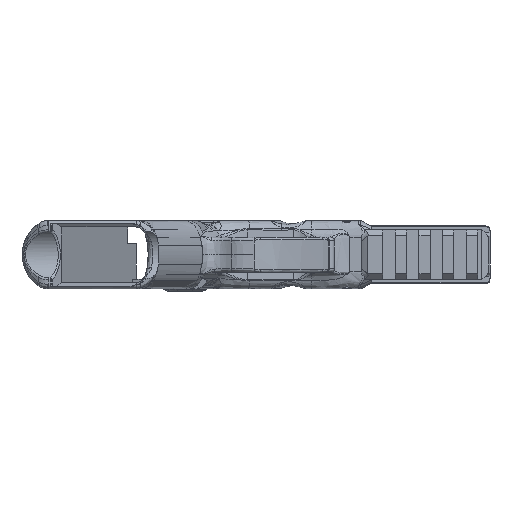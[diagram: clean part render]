
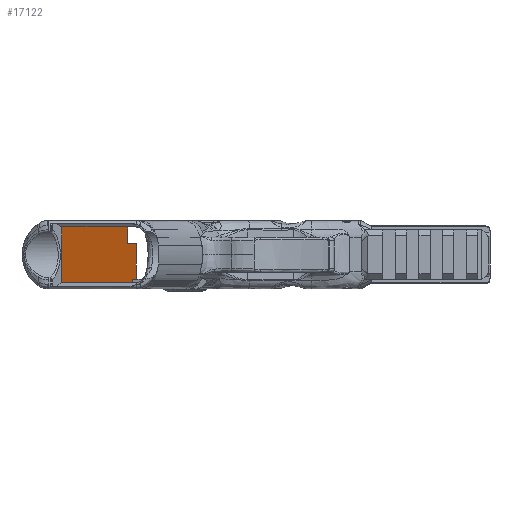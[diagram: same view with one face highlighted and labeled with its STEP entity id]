
A CAD part, front view. The second image highlights one B-rep face of the part: STEP entity #17122.
In plain terms, the highlighted planar face has unit normal (0.951, -0.309, 0).
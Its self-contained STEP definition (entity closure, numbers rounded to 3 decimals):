
#207 = ORIENTED_EDGE ( 'NONE', *, *, #1943, .F. ) ;
#595 = CARTESIAN_POINT ( 'NONE',  ( 2.237, -97.997, -11.765 ) ) ;
#730 = EDGE_CURVE ( 'NONE', #10152, #47471, #28344, .T. ) ;
#1692 = CARTESIAN_POINT ( 'NONE',  ( 33.591, -1.5, 4.75 ) ) ;
#1943 = EDGE_CURVE ( 'NONE', #28863, #14634, #2948, .T. ) ;
#2087 = CARTESIAN_POINT ( 'NONE',  ( 33.591, -1.5, -5.875 ) ) ;
#2320 = CARTESIAN_POINT ( 'NONE',  ( 18.86, -46.836, 4.75 ) ) ;
#2919 = CARTESIAN_POINT ( 'NONE',  ( 32.169, -5.875, -10.375 ) ) ;
#2948 =( BOUNDED_CURVE ( )  B_SPLINE_CURVE ( 3, ( #43225, #15098, #47478, #41535 ),
 .UNSPECIFIED., .F., .F. ) 
 B_SPLINE_CURVE_WITH_KNOTS ( ( 4, 4 ),
 ( 1.395, 1.571 ),
 .UNSPECIFIED. ) 
 CURVE ( )  GEOMETRIC_REPRESENTATION_ITEM ( )  RATIONAL_B_SPLINE_CURVE ( ( 1., 0.997, 0.997, 1. ) ) 
 REPRESENTATION_ITEM ( '' )  );
#3524 = DIRECTION ( 'NONE',  ( -0.951, 0.309, 0. ) ) ;
#3628 = VERTEX_POINT ( 'NONE', #1692 ) ;
#5233 = VECTOR ( 'NONE', #49592, 1000. ) ;
#6991 = PLANE ( 'NONE',  #35532 ) ;
#7092 = VECTOR ( 'NONE', #26142, 1000. ) ;
#7588 = VECTOR ( 'NONE', #37738, 1000. ) ;
#7966 = CARTESIAN_POINT ( 'NONE',  ( 32.169, -5.875, -11.75 ) ) ;
#8550 = CARTESIAN_POINT ( 'NONE',  ( 2.256, -97.94, -11.755 ) ) ;
#8653 =( BOUNDED_CURVE ( )  B_SPLINE_CURVE ( 3, ( #23826, #12148, #40541, #45031 ),
 .UNSPECIFIED., .F., .F. ) 
 B_SPLINE_CURVE_WITH_KNOTS ( ( 4, 4 ),
 ( 4.888, 4.891 ),
 .UNSPECIFIED. ) 
 CURVE ( )  GEOMETRIC_REPRESENTATION_ITEM ( )  RATIONAL_B_SPLINE_CURVE ( ( 1., 1., 1., 1. ) ) 
 REPRESENTATION_ITEM ( '' )  );
#10152 = VERTEX_POINT ( 'NONE', #47347 ) ;
#10278 = LINE ( 'NONE', #2087, #29029 ) ;
#10696 = LINE ( 'NONE', #39086, #15399 ) ;
#10897 = ORIENTED_EDGE ( 'NONE', *, *, #45271, .T. ) ;
#10984 = VERTEX_POINT ( 'NONE', #22116 ) ;
#12148 = CARTESIAN_POINT ( 'NONE',  ( 2.236, -97.998, -11.766 ) ) ;
#13134 = LINE ( 'NONE', #41264, #7092 ) ;
#13365 = EDGE_CURVE ( 'NONE', #47471, #16325, #8653, .T. ) ;
#13889 =( BOUNDED_CURVE ( )  B_SPLINE_CURVE ( 3, ( #15627, #19864, #15879, #28092 ),
 .UNSPECIFIED., .F., .T. ) 
 B_SPLINE_CURVE_WITH_KNOTS ( ( 4, 4 ),
 ( 1.392, 1.395 ),
 .UNSPECIFIED. ) 
 CURVE ( )  GEOMETRIC_REPRESENTATION_ITEM ( )  RATIONAL_B_SPLINE_CURVE ( ( 1., 1., 1., 1. ) ) 
 REPRESENTATION_ITEM ( '' )  );
#14178 = CARTESIAN_POINT ( 'NONE',  ( 2.237, -97.997, 11.765 ) ) ;
#14406 = DIRECTION ( 'NONE',  ( 0.309, 0.951, 0. ) ) ;
#14634 = VERTEX_POINT ( 'NONE', #44199 ) ;
#14932 = LINE ( 'NONE', #27139, #17959 ) ;
#15098 = CARTESIAN_POINT ( 'NONE',  ( 2.256, -97.94, 11.755 ) ) ;
#15399 = VECTOR ( 'NONE', #30874, 1000. ) ;
#15627 = CARTESIAN_POINT ( 'NONE',  ( 2.236, -98., 11.766 ) ) ;
#15879 = CARTESIAN_POINT ( 'NONE',  ( 2.236, -97.998, 11.766 ) ) ;
#16325 = VERTEX_POINT ( 'NONE', #28837 ) ;
#17122 = ADVANCED_FACE ( 'NONE', ( #27162 ), #6991, .F. ) ;
#17355 = EDGE_CURVE ( 'NONE', #42241, #39811, #38516, .T. ) ;
#17841 = EDGE_CURVE ( 'NONE', #16325, #31457, #30119, .T. ) ;
#17959 = VECTOR ( 'NONE', #14406, 1000. ) ;
#19864 = CARTESIAN_POINT ( 'NONE',  ( 2.236, -97.999, 11.766 ) ) ;
#20340 = EDGE_CURVE ( 'NONE', #3628, #10984, #10278, .T. ) ;
#20362 = EDGE_LOOP ( 'NONE', ( #10897, #207, #41972, #41069, #48009, #37743, #21009, #44787, #26066, #32704, #47489, #22947 ) ) ;
#21003 = VERTEX_POINT ( 'NONE', #7966 ) ;
#21009 = ORIENTED_EDGE ( 'NONE', *, *, #26845, .T. ) ;
#22116 = CARTESIAN_POINT ( 'NONE',  ( 33.591, -1.5, -10.375 ) ) ;
#22924 = DIRECTION ( 'NONE',  ( 0., 0., 1. ) ) ;
#22947 = ORIENTED_EDGE ( 'NONE', *, *, #17355, .F. ) ;
#23177 = DIRECTION ( 'NONE',  ( 0., 0., 1. ) ) ;
#23681 = CARTESIAN_POINT ( 'NONE',  ( 2.312, -97.765, -11.75 ) ) ;
#23826 = CARTESIAN_POINT ( 'NONE',  ( 2.237, -97.997, -11.765 ) ) ;
#24231 = CARTESIAN_POINT ( 'NONE',  ( 2.274, -97.881, -11.75 ) ) ;
#24253 = CARTESIAN_POINT ( 'NONE',  ( 30.049, -12.4, 11.75 ) ) ;
#24486 = CARTESIAN_POINT ( 'NONE',  ( 2.294, -97.822, -11.75 ) ) ;
#26066 = ORIENTED_EDGE ( 'NONE', *, *, #28083, .F. ) ;
#26142 = DIRECTION ( 'NONE',  ( -0.309, -0.951, 0. ) ) ;
#26670 = CARTESIAN_POINT ( 'NONE',  ( 2.236, -98., -18.375 ) ) ;
#26845 = EDGE_CURVE ( 'NONE', #10152, #21003, #14932, .T. ) ;
#27017 = DIRECTION ( 'NONE',  ( 0., 0., -1. ) ) ;
#27139 = CARTESIAN_POINT ( 'NONE',  ( 2.312, -97.765, -11.75 ) ) ;
#27162 = FACE_OUTER_BOUND ( 'NONE', #20362, .T. ) ;
#27503 = EDGE_CURVE ( 'NONE', #37545, #21003, #10696, .T. ) ;
#28083 = EDGE_CURVE ( 'NONE', #10984, #37545, #50114, .T. ) ;
#28092 = CARTESIAN_POINT ( 'NONE',  ( 2.237, -97.997, 11.765 ) ) ;
#28344 =( BOUNDED_CURVE ( )  B_SPLINE_CURVE ( 3, ( #24486, #24231, #8550, #595 ),
 .UNSPECIFIED., .F., .F. ) 
 B_SPLINE_CURVE_WITH_KNOTS ( ( 4, 4 ),
 ( 4.712, 4.888 ),
 .UNSPECIFIED. ) 
 CURVE ( )  GEOMETRIC_REPRESENTATION_ITEM ( )  RATIONAL_B_SPLINE_CURVE ( ( 1., 0.997, 0.997, 1. ) ) 
 REPRESENTATION_ITEM ( '' )  );
#28837 = CARTESIAN_POINT ( 'NONE',  ( 2.236, -98., -11.766 ) ) ;
#28863 = VERTEX_POINT ( 'NONE', #14178 ) ;
#29029 = VECTOR ( 'NONE', #27017, 1000. ) ;
#29960 = CARTESIAN_POINT ( 'NONE',  ( 2.237, -97.997, -11.765 ) ) ;
#29965 = CARTESIAN_POINT ( 'NONE',  ( 17.241, -51.82, -10.375 ) ) ;
#30119 = LINE ( 'NONE', #26670, #46768 ) ;
#30817 = CARTESIAN_POINT ( 'NONE',  ( 30.049, -12.4, 2.982 ) ) ;
#30874 = DIRECTION ( 'NONE',  ( 0., 0., -1. ) ) ;
#31457 = VERTEX_POINT ( 'NONE', #35554 ) ;
#32704 = ORIENTED_EDGE ( 'NONE', *, *, #20340, .F. ) ;
#33811 = CARTESIAN_POINT ( 'NONE',  ( 30.049, -12.4, 4.75 ) ) ;
#35532 = AXIS2_PLACEMENT_3D ( 'NONE', #23681, #3524, #23177 ) ;
#35554 = CARTESIAN_POINT ( 'NONE',  ( 2.236, -98., 11.766 ) ) ;
#37545 = VERTEX_POINT ( 'NONE', #2919 ) ;
#37647 = EDGE_CURVE ( 'NONE', #31457, #28863, #13889, .T. ) ;
#37738 = DIRECTION ( 'NONE',  ( 0., 0., -1. ) ) ;
#37743 = ORIENTED_EDGE ( 'NONE', *, *, #730, .F. ) ;
#38516 = LINE ( 'NONE', #30817, #7588 ) ;
#39086 = CARTESIAN_POINT ( 'NONE',  ( 32.169, -5.875, -5.875 ) ) ;
#39811 = VERTEX_POINT ( 'NONE', #33811 ) ;
#40541 = CARTESIAN_POINT ( 'NONE',  ( 2.236, -97.999, -11.766 ) ) ;
#41069 = ORIENTED_EDGE ( 'NONE', *, *, #17841, .F. ) ;
#41264 = CARTESIAN_POINT ( 'NONE',  ( 2.312, -97.765, 11.75 ) ) ;
#41535 = CARTESIAN_POINT ( 'NONE',  ( 2.294, -97.822, 11.75 ) ) ;
#41972 = ORIENTED_EDGE ( 'NONE', *, *, #37647, .F. ) ;
#42241 = VERTEX_POINT ( 'NONE', #24253 ) ;
#42894 = DIRECTION ( 'NONE',  ( 0.309, 0.951, 0. ) ) ;
#43225 = CARTESIAN_POINT ( 'NONE',  ( 2.237, -97.997, 11.765 ) ) ;
#44199 = CARTESIAN_POINT ( 'NONE',  ( 2.294, -97.822, 11.75 ) ) ;
#44787 = ORIENTED_EDGE ( 'NONE', *, *, #27503, .F. ) ;
#44968 = EDGE_CURVE ( 'NONE', #39811, #3628, #47405, .T. ) ;
#45031 = CARTESIAN_POINT ( 'NONE',  ( 2.236, -98., -11.766 ) ) ;
#45271 = EDGE_CURVE ( 'NONE', #42241, #14634, #13134, .T. ) ;
#46768 = VECTOR ( 'NONE', #22924, 1000. ) ;
#47347 = CARTESIAN_POINT ( 'NONE',  ( 2.294, -97.822, -11.75 ) ) ;
#47405 = LINE ( 'NONE', #2320, #47751 ) ;
#47471 = VERTEX_POINT ( 'NONE', #29960 ) ;
#47478 = CARTESIAN_POINT ( 'NONE',  ( 2.274, -97.881, 11.75 ) ) ;
#47489 = ORIENTED_EDGE ( 'NONE', *, *, #44968, .F. ) ;
#47751 = VECTOR ( 'NONE', #42894, 1000. ) ;
#48009 = ORIENTED_EDGE ( 'NONE', *, *, #13365, .F. ) ;
#49592 = DIRECTION ( 'NONE',  ( -0.309, -0.951, 0. ) ) ;
#50114 = LINE ( 'NONE', #29965, #5233 ) ;
